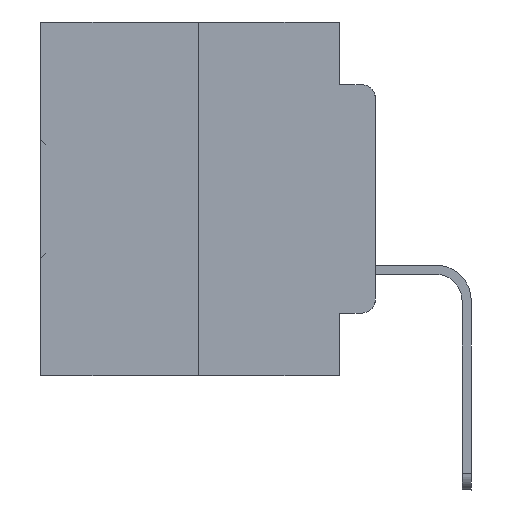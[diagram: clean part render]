
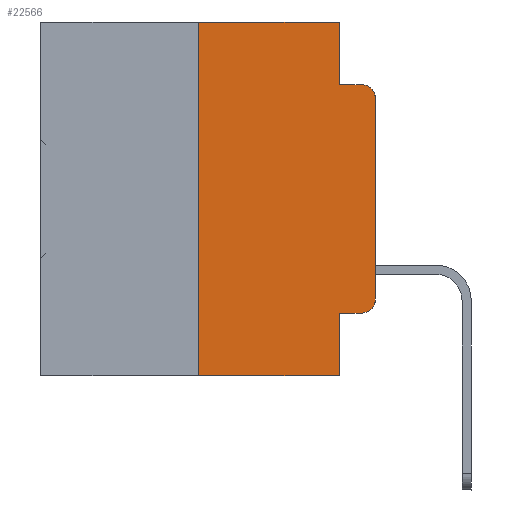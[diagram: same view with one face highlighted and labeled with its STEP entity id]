
A CAD part, left-side view. The second image highlights one B-rep face of the part: STEP entity #22566.
In plain terms, the highlighted planar face has unit normal (-1, 0, 0).
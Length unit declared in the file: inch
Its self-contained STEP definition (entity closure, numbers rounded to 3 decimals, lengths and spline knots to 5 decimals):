
#218 = DIRECTION ( 'NONE',  ( 1., 0., 0. ) ) ;
#841 = CARTESIAN_POINT ( 'NONE',  ( 0., 0.051, 0. ) ) ;
#1008 = CIRCLE ( 'NONE', #11787, 0.02 ) ;
#1448 = VECTOR ( 'NONE', #17955, 39.37008 ) ;
#1995 = CARTESIAN_POINT ( 'NONE',  ( 0., 0.02, -0.4115 ) ) ;
#2036 = CARTESIAN_POINT ( 'NONE',  ( 0., 0.051, 0. ) ) ;
#2751 = CARTESIAN_POINT ( 'NONE',  ( 0., 0.473, -0.5 ) ) ;
#2872 = CARTESIAN_POINT ( 'NONE',  ( 0., 0., -0.3915 ) ) ;
#3882 = VERTEX_POINT ( 'NONE', #10967 ) ;
#4014 = VECTOR ( 'NONE', #11570, 39.37008 ) ;
#4251 = ORIENTED_EDGE ( 'NONE', *, *, #23879, .F. ) ;
#4373 = VECTOR ( 'NONE', #13875, 39.37008 ) ;
#4542 = ORIENTED_EDGE ( 'NONE', *, *, #21433, .F. ) ;
#4671 = CARTESIAN_POINT ( 'NONE',  ( 0., 0.02, -0.1085 ) ) ;
#5262 = LINE ( 'NONE', #14286, #4014 ) ;
#5824 = LINE ( 'NONE', #22639, #28367 ) ;
#6602 = ORIENTED_EDGE ( 'NONE', *, *, #12090, .T. ) ;
#7543 = VERTEX_POINT ( 'NONE', #9201 ) ;
#7701 = VERTEX_POINT ( 'NONE', #25784 ) ;
#7731 = ORIENTED_EDGE ( 'NONE', *, *, #22275, .T. ) ;
#7850 = DIRECTION ( 'NONE',  ( 0., -1., 0. ) ) ;
#7953 = LINE ( 'NONE', #29938, #11322 ) ;
#8374 = PLANE ( 'NONE',  #17014 ) ;
#9201 = CARTESIAN_POINT ( 'NONE',  ( 0., 0.051, -0.0885 ) ) ;
#9595 = EDGE_LOOP ( 'NONE', ( #34414, #7731, #16694, #4542, #4251, #13745, #15206, #28081, #6602, #17907 ) ) ;
#10719 = DIRECTION ( 'NONE',  ( 0., 0., -1. ) ) ;
#10967 = CARTESIAN_POINT ( 'NONE',  ( 0., 0.25, 0. ) ) ;
#11322 = VECTOR ( 'NONE', #16769, 39.37008 ) ;
#11570 = DIRECTION ( 'NONE',  ( 0., 0., 1. ) ) ;
#11696 = EDGE_CURVE ( 'NONE', #7701, #31856, #12307, .T. ) ;
#11787 = AXIS2_PLACEMENT_3D ( 'NONE', #4671, #23235, #14994 ) ;
#12090 = EDGE_CURVE ( 'NONE', #7701, #25966, #5824, .T. ) ;
#12307 = LINE ( 'NONE', #2036, #1448 ) ;
#13140 = CIRCLE ( 'NONE', #20859, 0.02 ) ;
#13155 = DIRECTION ( 'NONE',  ( 0., -1., 0. ) ) ;
#13745 = ORIENTED_EDGE ( 'NONE', *, *, #25270, .F. ) ;
#13875 = DIRECTION ( 'NONE',  ( 0., 0., -1. ) ) ;
#14260 = DIRECTION ( 'NONE',  ( -1., 0., 0. ) ) ;
#14286 = CARTESIAN_POINT ( 'NONE',  ( 0., 0., 0. ) ) ;
#14994 = DIRECTION ( 'NONE',  ( 0., 0., -1. ) ) ;
#15206 = ORIENTED_EDGE ( 'NONE', *, *, #21314, .T. ) ;
#16328 = CARTESIAN_POINT ( 'NONE',  ( 0., 0., -0.1085 ) ) ;
#16535 = EDGE_CURVE ( 'NONE', #7543, #22167, #25251, .T. ) ;
#16694 = ORIENTED_EDGE ( 'NONE', *, *, #16535, .F. ) ;
#16769 = DIRECTION ( 'NONE',  ( 0., -1., 0. ) ) ;
#17014 = AXIS2_PLACEMENT_3D ( 'NONE', #18937, #218, #10719 ) ;
#17592 = CARTESIAN_POINT ( 'NONE',  ( 0., 0.25, -0.5 ) ) ;
#17907 = ORIENTED_EDGE ( 'NONE', *, *, #31660, .T. ) ;
#17955 = DIRECTION ( 'NONE',  ( 0., 0., -1. ) ) ;
#18172 = VECTOR ( 'NONE', #7850, 39.37008 ) ;
#18626 = LINE ( 'NONE', #2751, #32811 ) ;
#18937 = CARTESIAN_POINT ( 'NONE',  ( 0., 0.473, 0. ) ) ;
#19031 = LINE ( 'NONE', #27057, #4373 ) ;
#19855 = DIRECTION ( 'NONE',  ( 0., -1., 0. ) ) ;
#19856 = VERTEX_POINT ( 'NONE', #2872 ) ;
#20183 = LINE ( 'NONE', #20505, #33535 ) ;
#20505 = CARTESIAN_POINT ( 'NONE',  ( 0., 0.25, 0. ) ) ;
#20647 = EDGE_CURVE ( 'NONE', #19856, #25538, #5262, .T. ) ;
#20859 = AXIS2_PLACEMENT_3D ( 'NONE', #21959, #14260, #32815 ) ;
#21314 = EDGE_CURVE ( 'NONE', #33069, #31856, #18626, .T. ) ;
#21433 = EDGE_CURVE ( 'NONE', #30858, #7543, #19031, .T. ) ;
#21532 = CARTESIAN_POINT ( 'NONE',  ( 0., 0.051, -0.0885 ) ) ;
#21959 = CARTESIAN_POINT ( 'NONE',  ( 0., 0.02, -0.3915 ) ) ;
#22167 = VERTEX_POINT ( 'NONE', #33415 ) ;
#22275 = EDGE_CURVE ( 'NONE', #25538, #22167, #1008, .T. ) ;
#22566 = ADVANCED_FACE ( 'NONE', ( #23110 ), #8374, .F. ) ;
#22639 = CARTESIAN_POINT ( 'NONE',  ( 0., 0.051, -0.4115 ) ) ;
#23110 = FACE_OUTER_BOUND ( 'NONE', #9595, .T. ) ;
#23204 = CARTESIAN_POINT ( 'NONE',  ( 0., 0.051, -0.5 ) ) ;
#23235 = DIRECTION ( 'NONE',  ( -1., 0., 0. ) ) ;
#23879 = EDGE_CURVE ( 'NONE', #3882, #30858, #7953, .T. ) ;
#25251 = LINE ( 'NONE', #21532, #18172 ) ;
#25270 = EDGE_CURVE ( 'NONE', #33069, #3882, #20183, .T. ) ;
#25538 = VERTEX_POINT ( 'NONE', #16328 ) ;
#25784 = CARTESIAN_POINT ( 'NONE',  ( 0., 0.051, -0.4115 ) ) ;
#25966 = VERTEX_POINT ( 'NONE', #1995 ) ;
#27057 = CARTESIAN_POINT ( 'NONE',  ( 0., 0.051, 0. ) ) ;
#28081 = ORIENTED_EDGE ( 'NONE', *, *, #11696, .F. ) ;
#28367 = VECTOR ( 'NONE', #19855, 39.37008 ) ;
#28777 = DIRECTION ( 'NONE',  ( 0., 0., 1. ) ) ;
#29938 = CARTESIAN_POINT ( 'NONE',  ( 0., 0.473, 0. ) ) ;
#30858 = VERTEX_POINT ( 'NONE', #841 ) ;
#31660 = EDGE_CURVE ( 'NONE', #25966, #19856, #13140, .T. ) ;
#31856 = VERTEX_POINT ( 'NONE', #23204 ) ;
#32811 = VECTOR ( 'NONE', #13155, 39.37008 ) ;
#32815 = DIRECTION ( 'NONE',  ( 0., 0., -1. ) ) ;
#33069 = VERTEX_POINT ( 'NONE', #17592 ) ;
#33415 = CARTESIAN_POINT ( 'NONE',  ( 0., 0.02, -0.0885 ) ) ;
#33535 = VECTOR ( 'NONE', #28777, 39.37008 ) ;
#34414 = ORIENTED_EDGE ( 'NONE', *, *, #20647, .T. ) ;
